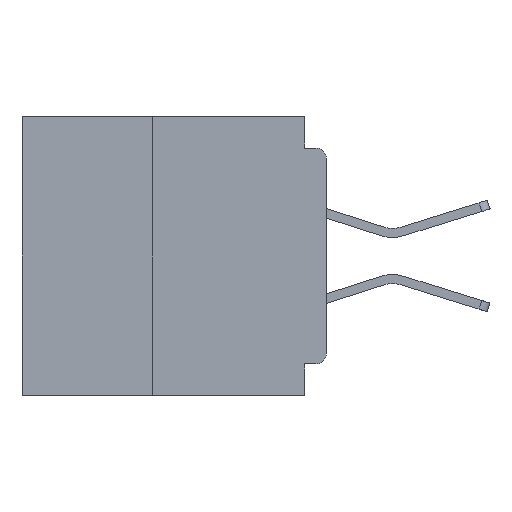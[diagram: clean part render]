
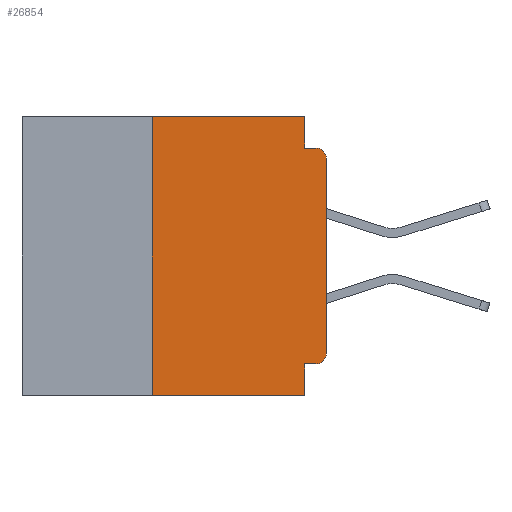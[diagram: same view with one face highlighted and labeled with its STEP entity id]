
A CAD part, left-side view. The second image highlights one B-rep face of the part: STEP entity #26854.
In plain terms, the highlighted planar face has unit normal (-1, 0, 0).
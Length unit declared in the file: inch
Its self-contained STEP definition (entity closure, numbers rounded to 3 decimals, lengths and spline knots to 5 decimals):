
#823 = ORIENTED_EDGE ( 'NONE', *, *, #3219, .T. ) ;
#1062 = DIRECTION ( 'NONE',  ( 0., 0., 1. ) ) ;
#1628 = EDGE_CURVE ( 'NONE', #30697, #23586, #21139, .T. ) ;
#1752 = CARTESIAN_POINT ( 'NONE',  ( 0., 0.437, 0. ) ) ;
#1912 = EDGE_CURVE ( 'NONE', #37599, #42057, #35528, .T. ) ;
#3219 = EDGE_CURVE ( 'NONE', #23586, #10022, #36060, .T. ) ;
#4275 = PLANE ( 'NONE',  #7791 ) ;
#4353 = ORIENTED_EDGE ( 'NONE', *, *, #31438, .F. ) ;
#4611 = DIRECTION ( 'NONE',  ( 1., 0., 0. ) ) ;
#4773 = DIRECTION ( 'NONE',  ( 0., -1., 0. ) ) ;
#5173 = VECTOR ( 'NONE', #38766, 39.37008 ) ;
#5809 = CARTESIAN_POINT ( 'NONE',  ( 0., 0.031, 0. ) ) ;
#6293 = LINE ( 'NONE', #19482, #16093 ) ;
#7012 = VECTOR ( 'NONE', #20410, 39.37008 ) ;
#7791 = AXIS2_PLACEMENT_3D ( 'NONE', #26818, #4611, #30502 ) ;
#8391 = CARTESIAN_POINT ( 'NONE',  ( 0., 0.031, -0.045 ) ) ;
#9149 = EDGE_CURVE ( 'NONE', #10022, #13685, #17074, .T. ) ;
#9237 = VERTEX_POINT ( 'NONE', #20649 ) ;
#10022 = VERTEX_POINT ( 'NONE', #39959 ) ;
#10100 = VERTEX_POINT ( 'NONE', #14764 ) ;
#11398 = VERTEX_POINT ( 'NONE', #11982 ) ;
#11982 = CARTESIAN_POINT ( 'NONE',  ( 0., 0.031, -0.355 ) ) ;
#12879 = CARTESIAN_POINT ( 'NONE',  ( 0., 0.015, -0.06 ) ) ;
#13685 = VERTEX_POINT ( 'NONE', #28323 ) ;
#14397 = VERTEX_POINT ( 'NONE', #41171 ) ;
#14764 = CARTESIAN_POINT ( 'NONE',  ( 0., 0.031, -0.4 ) ) ;
#15867 = CARTESIAN_POINT ( 'NONE',  ( 0., 0.25, -0.4 ) ) ;
#15884 = EDGE_CURVE ( 'NONE', #9237, #37599, #17969, .T. ) ;
#15916 = VECTOR ( 'NONE', #1062, 39.37008 ) ;
#15980 = ORIENTED_EDGE ( 'NONE', *, *, #1628, .T. ) ;
#16093 = VECTOR ( 'NONE', #4773, 39.37008 ) ;
#16165 = LINE ( 'NONE', #16459, #5173 ) ;
#16459 = CARTESIAN_POINT ( 'NONE',  ( 0., 0., -0.355 ) ) ;
#16572 = EDGE_CURVE ( 'NONE', #30697, #11398, #16165, .T. ) ;
#16597 = DIRECTION ( 'NONE',  ( 0., 0., -1. ) ) ;
#17074 = CIRCLE ( 'NONE', #42630, 0.015 ) ;
#17431 = LINE ( 'NONE', #42508, #45565 ) ;
#17969 = LINE ( 'NONE', #1752, #7012 ) ;
#18723 = CARTESIAN_POINT ( 'NONE',  ( 0., 0., -0.34 ) ) ;
#19482 = CARTESIAN_POINT ( 'NONE',  ( 0., 0., -0.045 ) ) ;
#20285 = LINE ( 'NONE', #35195, #32399 ) ;
#20410 = DIRECTION ( 'NONE',  ( 0., -1., 0. ) ) ;
#20649 = CARTESIAN_POINT ( 'NONE',  ( 0., 0.25, 0. ) ) ;
#21139 = CIRCLE ( 'NONE', #34431, 0.015 ) ;
#22815 = DIRECTION ( 'NONE',  ( 0., 0., -1. ) ) ;
#23586 = VERTEX_POINT ( 'NONE', #18723 ) ;
#24281 = CARTESIAN_POINT ( 'NONE',  ( 0., 0.031, 0. ) ) ;
#24705 = ORIENTED_EDGE ( 'NONE', *, *, #16572, .F. ) ;
#24724 = FACE_OUTER_BOUND ( 'NONE', #31884, .T. ) ;
#25788 = LINE ( 'NONE', #15867, #15916 ) ;
#26818 = CARTESIAN_POINT ( 'NONE',  ( 0., 0.437, 0. ) ) ;
#26854 = ADVANCED_FACE ( 'NONE', ( #24724 ), #4275, .F. ) ;
#28323 = CARTESIAN_POINT ( 'NONE',  ( 0., 0.015, -0.045 ) ) ;
#28721 = ORIENTED_EDGE ( 'NONE', *, *, #44853, .F. ) ;
#30502 = DIRECTION ( 'NONE',  ( 0., 0., -1. ) ) ;
#30697 = VERTEX_POINT ( 'NONE', #37625 ) ;
#31006 = ORIENTED_EDGE ( 'NONE', *, *, #40079, .T. ) ;
#31438 = EDGE_CURVE ( 'NONE', #42057, #13685, #6293, .T. ) ;
#31490 = DIRECTION ( 'NONE',  ( 0., 0., -1. ) ) ;
#31884 = EDGE_LOOP ( 'NONE', ( #823, #40212, #4353, #33836, #45813, #28721, #31006, #41920, #24705, #15980 ) ) ;
#32399 = VECTOR ( 'NONE', #31490, 39.37008 ) ;
#33836 = ORIENTED_EDGE ( 'NONE', *, *, #1912, .F. ) ;
#34431 = AXIS2_PLACEMENT_3D ( 'NONE', #41163, #40968, #40854 ) ;
#35149 = DIRECTION ( 'NONE',  ( 0., -1., 0. ) ) ;
#35195 = CARTESIAN_POINT ( 'NONE',  ( 0., 0.031, -0.4 ) ) ;
#35528 = LINE ( 'NONE', #24281, #44042 ) ;
#36060 = LINE ( 'NONE', #47188, #45693 ) ;
#37586 = EDGE_CURVE ( 'NONE', #11398, #10100, #20285, .T. ) ;
#37599 = VERTEX_POINT ( 'NONE', #5809 ) ;
#37625 = CARTESIAN_POINT ( 'NONE',  ( 0., 0.015, -0.355 ) ) ;
#38741 = DIRECTION ( 'NONE',  ( -1., 0., 0. ) ) ;
#38766 = DIRECTION ( 'NONE',  ( 0., 1., 0. ) ) ;
#39959 = CARTESIAN_POINT ( 'NONE',  ( 0., 0., -0.06 ) ) ;
#40079 = EDGE_CURVE ( 'NONE', #14397, #10100, #17431, .T. ) ;
#40212 = ORIENTED_EDGE ( 'NONE', *, *, #9149, .T. ) ;
#40854 = DIRECTION ( 'NONE',  ( 0., 0., -1. ) ) ;
#40968 = DIRECTION ( 'NONE',  ( -1., 0., 0. ) ) ;
#41163 = CARTESIAN_POINT ( 'NONE',  ( 0., 0.015, -0.34 ) ) ;
#41171 = CARTESIAN_POINT ( 'NONE',  ( 0., 0.25, -0.4 ) ) ;
#41920 = ORIENTED_EDGE ( 'NONE', *, *, #37586, .F. ) ;
#42057 = VERTEX_POINT ( 'NONE', #8391 ) ;
#42508 = CARTESIAN_POINT ( 'NONE',  ( 0., 0.437, -0.4 ) ) ;
#42630 = AXIS2_PLACEMENT_3D ( 'NONE', #12879, #38741, #16597 ) ;
#44042 = VECTOR ( 'NONE', #22815, 39.37008 ) ;
#44853 = EDGE_CURVE ( 'NONE', #14397, #9237, #25788, .T. ) ;
#45565 = VECTOR ( 'NONE', #35149, 39.37008 ) ;
#45693 = VECTOR ( 'NONE', #47354, 39.37008 ) ;
#45813 = ORIENTED_EDGE ( 'NONE', *, *, #15884, .F. ) ;
#47188 = CARTESIAN_POINT ( 'NONE',  ( 0., 0., 0. ) ) ;
#47354 = DIRECTION ( 'NONE',  ( 0., 0., 1. ) ) ;
